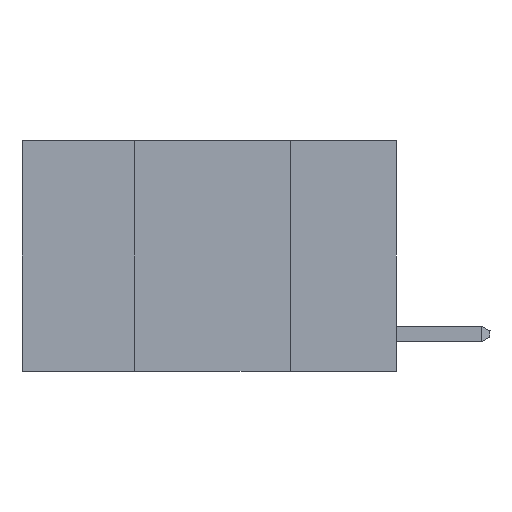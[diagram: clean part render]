
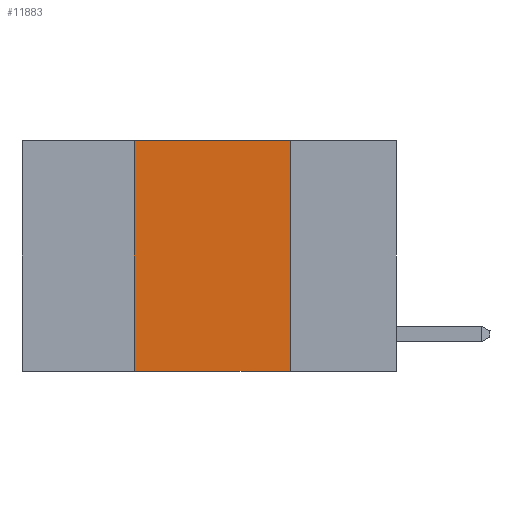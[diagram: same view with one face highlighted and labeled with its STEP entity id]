
A CAD part, left-side view. The second image highlights one B-rep face of the part: STEP entity #11883.
In plain terms, the highlighted planar face has unit normal (-1, 0, 0).
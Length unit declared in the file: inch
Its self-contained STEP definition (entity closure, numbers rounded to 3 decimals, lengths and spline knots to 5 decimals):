
#352 = VECTOR ( 'NONE', #13383, 39.37008 ) ;
#1096 = ORIENTED_EDGE ( 'NONE', *, *, #5588, .F. ) ;
#3065 = LINE ( 'NONE', #10718, #3669 ) ;
#3551 = CARTESIAN_POINT ( 'NONE',  ( 0., 0.42, 0. ) ) ;
#3597 = EDGE_LOOP ( 'NONE', ( #10083, #1096, #11255, #16553 ) ) ;
#3669 = VECTOR ( 'NONE', #13531, 39.37008 ) ;
#4513 = VERTEX_POINT ( 'NONE', #7042 ) ;
#4916 = PLANE ( 'NONE',  #6809 ) ;
#4991 = DIRECTION ( 'NONE',  ( 0., -1., 0. ) ) ;
#5086 = DIRECTION ( 'NONE',  ( 1., 0., 0. ) ) ;
#5229 = CARTESIAN_POINT ( 'NONE',  ( 0., 0.6, -0.37 ) ) ;
#5305 = VERTEX_POINT ( 'NONE', #3551 ) ;
#5409 = VECTOR ( 'NONE', #12010, 39.37008 ) ;
#5580 = VECTOR ( 'NONE', #4991, 39.37008 ) ;
#5588 = EDGE_CURVE ( 'NONE', #5305, #14809, #12385, .T. ) ;
#6809 = AXIS2_PLACEMENT_3D ( 'NONE', #9949, #5086, #14200 ) ;
#6857 = EDGE_CURVE ( 'NONE', #9350, #4513, #12577, .T. ) ;
#7042 = CARTESIAN_POINT ( 'NONE',  ( 0., 0.17, -0.37 ) ) ;
#7570 = CARTESIAN_POINT ( 'NONE',  ( 0., 0.42, -0.37 ) ) ;
#8147 = FACE_OUTER_BOUND ( 'NONE', #3597, .T. ) ;
#9330 = LINE ( 'NONE', #13232, #5409 ) ;
#9350 = VERTEX_POINT ( 'NONE', #7570 ) ;
#9949 = CARTESIAN_POINT ( 'NONE',  ( 0., 0.6, 0. ) ) ;
#10083 = ORIENTED_EDGE ( 'NONE', *, *, #11691, .F. ) ;
#10718 = CARTESIAN_POINT ( 'NONE',  ( 0., 0.42, 0. ) ) ;
#11255 = ORIENTED_EDGE ( 'NONE', *, *, #16684, .F. ) ;
#11691 = EDGE_CURVE ( 'NONE', #14809, #4513, #9330, .T. ) ;
#11883 = ADVANCED_FACE ( 'NONE', ( #8147 ), #4916, .F. ) ;
#12010 = DIRECTION ( 'NONE',  ( 0., 0., -1. ) ) ;
#12385 = LINE ( 'NONE', #14704, #352 ) ;
#12577 = LINE ( 'NONE', #5229, #5580 ) ;
#13232 = CARTESIAN_POINT ( 'NONE',  ( 0., 0.17, 0. ) ) ;
#13383 = DIRECTION ( 'NONE',  ( 0., -1., 0. ) ) ;
#13531 = DIRECTION ( 'NONE',  ( 0., 0., 1. ) ) ;
#14200 = DIRECTION ( 'NONE',  ( 0., 0., -1. ) ) ;
#14704 = CARTESIAN_POINT ( 'NONE',  ( 0., 0.6, 0. ) ) ;
#14809 = VERTEX_POINT ( 'NONE', #16800 ) ;
#16553 = ORIENTED_EDGE ( 'NONE', *, *, #6857, .T. ) ;
#16684 = EDGE_CURVE ( 'NONE', #9350, #5305, #3065, .T. ) ;
#16800 = CARTESIAN_POINT ( 'NONE',  ( 0., 0.17, 0. ) ) ;
